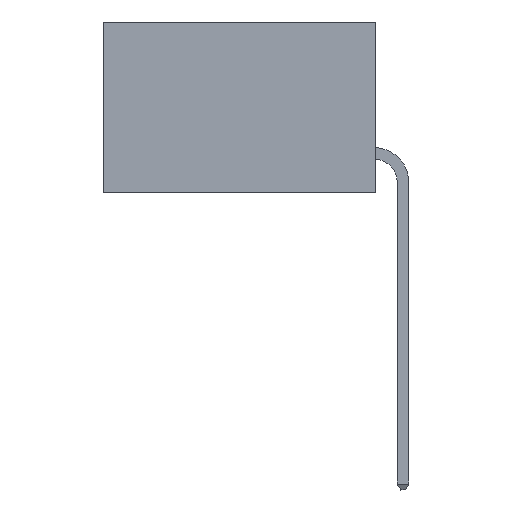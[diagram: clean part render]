
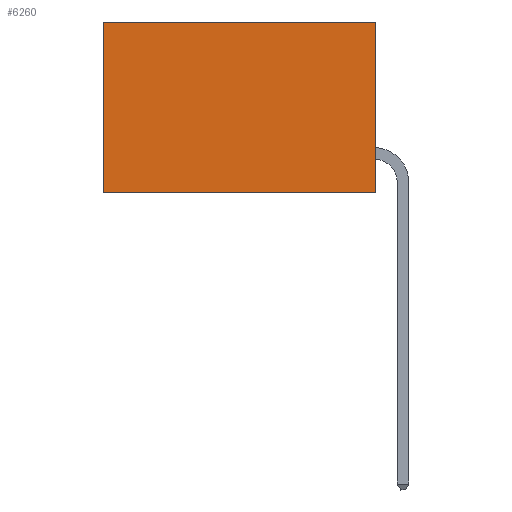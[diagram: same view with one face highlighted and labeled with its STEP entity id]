
A CAD part, left-side view. The second image highlights one B-rep face of the part: STEP entity #6260.
In plain terms, the highlighted planar face has unit normal (-1, 0, 0).
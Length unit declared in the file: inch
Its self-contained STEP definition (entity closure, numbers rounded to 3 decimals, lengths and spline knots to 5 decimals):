
#369 = CARTESIAN_POINT ( 'NONE',  ( 0.277, 0., -0.37 ) ) ;
#681 = LINE ( 'NONE', #5810, #9393 ) ;
#695 = CARTESIAN_POINT ( 'NONE',  ( 0.277, 0., -0.37 ) ) ;
#2147 = VERTEX_POINT ( 'NONE', #11325 ) ;
#2601 = VECTOR ( 'NONE', #4968, 39.37008 ) ;
#3609 = VERTEX_POINT ( 'NONE', #369 ) ;
#4317 = ORIENTED_EDGE ( 'NONE', *, *, #5069, .F. ) ;
#4466 = FACE_OUTER_BOUND ( 'NONE', #13754, .T. ) ;
#4795 = ORIENTED_EDGE ( 'NONE', *, *, #6229, .T. ) ;
#4968 = DIRECTION ( 'NONE',  ( 0., 1., 0. ) ) ;
#5019 = EDGE_CURVE ( 'NONE', #3609, #7338, #8616, .T. ) ;
#5069 = EDGE_CURVE ( 'NONE', #2147, #3609, #8282, .T. ) ;
#5250 = DIRECTION ( 'NONE',  ( 0., 0., -1. ) ) ;
#5287 = DIRECTION ( 'NONE',  ( 1., 0., 0. ) ) ;
#5369 = PLANE ( 'NONE',  #6729 ) ;
#5424 = CARTESIAN_POINT ( 'NONE',  ( 0.277, 0., -0.37 ) ) ;
#5598 = DIRECTION ( 'NONE',  ( 0., 1., 0. ) ) ;
#5810 = CARTESIAN_POINT ( 'NONE',  ( 0.277, 0.59, -0.37 ) ) ;
#5876 = CARTESIAN_POINT ( 'NONE',  ( 0.277, 0.59, 0. ) ) ;
#5890 = CARTESIAN_POINT ( 'NONE',  ( 0.277, 0., 0. ) ) ;
#6225 = VERTEX_POINT ( 'NONE', #5876 ) ;
#6229 = EDGE_CURVE ( 'NONE', #2147, #6225, #8115, .T. ) ;
#6260 = ADVANCED_FACE ( 'NONE', ( #4466 ), #5369, .F. ) ;
#6729 = AXIS2_PLACEMENT_3D ( 'NONE', #5424, #5287, #5250 ) ;
#6895 = DIRECTION ( 'NONE',  ( 0., 0., -1. ) ) ;
#6999 = DIRECTION ( 'NONE',  ( 0., 0., -1. ) ) ;
#7338 = VERTEX_POINT ( 'NONE', #12355 ) ;
#7432 = ORIENTED_EDGE ( 'NONE', *, *, #5019, .F. ) ;
#8115 = LINE ( 'NONE', #5890, #13625 ) ;
#8282 = LINE ( 'NONE', #9889, #13462 ) ;
#8616 = LINE ( 'NONE', #695, #2601 ) ;
#9393 = VECTOR ( 'NONE', #6999, 39.37008 ) ;
#9889 = CARTESIAN_POINT ( 'NONE',  ( 0.277, 0., -0.37 ) ) ;
#11325 = CARTESIAN_POINT ( 'NONE',  ( 0.277, 0., 0. ) ) ;
#12255 = EDGE_CURVE ( 'NONE', #6225, #7338, #681, .T. ) ;
#12355 = CARTESIAN_POINT ( 'NONE',  ( 0.277, 0.59, -0.37 ) ) ;
#13196 = ORIENTED_EDGE ( 'NONE', *, *, #12255, .T. ) ;
#13462 = VECTOR ( 'NONE', #6895, 39.37008 ) ;
#13625 = VECTOR ( 'NONE', #5598, 39.37008 ) ;
#13754 = EDGE_LOOP ( 'NONE', ( #13196, #7432, #4317, #4795 ) ) ;
